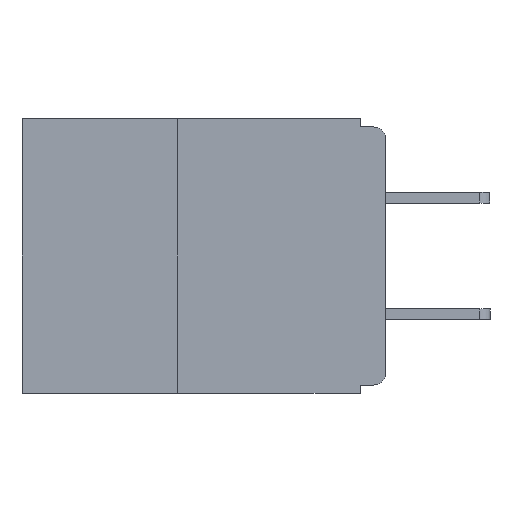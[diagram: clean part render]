
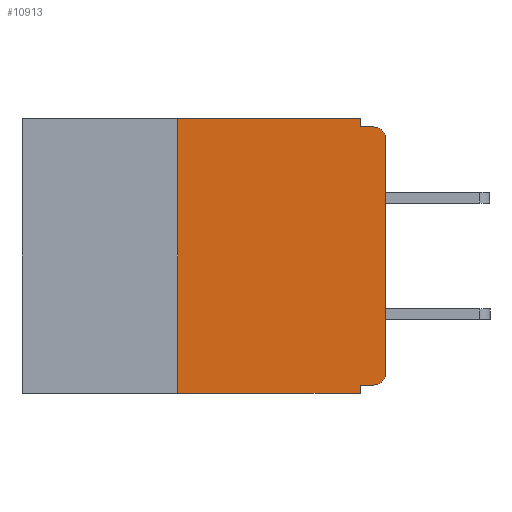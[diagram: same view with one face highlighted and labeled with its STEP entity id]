
A CAD part, left-side view. The second image highlights one B-rep face of the part: STEP entity #10913.
In plain terms, the highlighted planar face has unit normal (-1, 0, 0).
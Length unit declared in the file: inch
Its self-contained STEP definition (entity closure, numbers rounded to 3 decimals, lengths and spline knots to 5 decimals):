
#455 = CARTESIAN_POINT ( 'NONE',  ( 0., 0.437, -0.33 ) ) ;
#553 = VERTEX_POINT ( 'NONE', #17320 ) ;
#639 = CARTESIAN_POINT ( 'NONE',  ( 0., 0., -0.01 ) ) ;
#657 = CARTESIAN_POINT ( 'NONE',  ( 0., 0., -0.025 ) ) ;
#842 = CARTESIAN_POINT ( 'NONE',  ( 0., 0.031, 0. ) ) ;
#1207 = DIRECTION ( 'NONE',  ( 0., 0., -1. ) ) ;
#1218 = DIRECTION ( 'NONE',  ( 0., 0., -1. ) ) ;
#2066 = VECTOR ( 'NONE', #16568, 39.37008 ) ;
#2387 = EDGE_CURVE ( 'NONE', #8167, #9338, #11004, .T. ) ;
#2638 = CARTESIAN_POINT ( 'NONE',  ( 0., 0.25, 0. ) ) ;
#2918 = FACE_OUTER_BOUND ( 'NONE', #9005, .T. ) ;
#2960 = DIRECTION ( 'NONE',  ( 0., 0., -1. ) ) ;
#2979 = VERTEX_POINT ( 'NONE', #2638 ) ;
#2989 = VECTOR ( 'NONE', #12892, 39.37008 ) ;
#3006 = DIRECTION ( 'NONE',  ( 1., 0., 0. ) ) ;
#3076 = CARTESIAN_POINT ( 'NONE',  ( 0., 0.437, 0. ) ) ;
#3279 = PLANE ( 'NONE',  #16611 ) ;
#3420 = CARTESIAN_POINT ( 'NONE',  ( 0., 0.015, -0.01 ) ) ;
#3581 = CARTESIAN_POINT ( 'NONE',  ( 0., 0.031, -0.01 ) ) ;
#3980 = CARTESIAN_POINT ( 'NONE',  ( 0., 0., 0. ) ) ;
#4009 = VECTOR ( 'NONE', #13741, 39.37008 ) ;
#4166 = LINE ( 'NONE', #3980, #15136 ) ;
#4281 = DIRECTION ( 'NONE',  ( 0., 0., -1. ) ) ;
#4480 = DIRECTION ( 'NONE',  ( 0., -1., 0. ) ) ;
#4575 = EDGE_CURVE ( 'NONE', #5898, #14512, #12701, .T. ) ;
#4947 = ORIENTED_EDGE ( 'NONE', *, *, #17764, .F. ) ;
#5235 = VERTEX_POINT ( 'NONE', #3581 ) ;
#5738 = CARTESIAN_POINT ( 'NONE',  ( 0., 0.015, -0.32 ) ) ;
#5811 = DIRECTION ( 'NONE',  ( 0., 0., 1. ) ) ;
#5898 = VERTEX_POINT ( 'NONE', #657 ) ;
#6132 = VERTEX_POINT ( 'NONE', #16183 ) ;
#6234 = DIRECTION ( 'NONE',  ( 0., 0., -1. ) ) ;
#6428 = EDGE_CURVE ( 'NONE', #8167, #2979, #15448, .T. ) ;
#6537 = DIRECTION ( 'NONE',  ( -1., 0., 0. ) ) ;
#6635 = CARTESIAN_POINT ( 'NONE',  ( 0., 0.015, -0.025 ) ) ;
#6837 = ORIENTED_EDGE ( 'NONE', *, *, #17963, .F. ) ;
#6995 = LINE ( 'NONE', #12105, #2989 ) ;
#7040 = ORIENTED_EDGE ( 'NONE', *, *, #4575, .T. ) ;
#7387 = EDGE_CURVE ( 'NONE', #6132, #5235, #10359, .T. ) ;
#7752 = ORIENTED_EDGE ( 'NONE', *, *, #8477, .F. ) ;
#8167 = VERTEX_POINT ( 'NONE', #14017 ) ;
#8477 = EDGE_CURVE ( 'NONE', #14852, #12403, #6995, .T. ) ;
#8780 = CARTESIAN_POINT ( 'NONE',  ( 0., 0.031, -0.33 ) ) ;
#8935 = AXIS2_PLACEMENT_3D ( 'NONE', #6635, #6537, #6234 ) ;
#9005 = EDGE_LOOP ( 'NONE', ( #17293, #7040, #4947, #15885, #13090, #13534, #17111, #6837, #7752, #15242 ) ) ;
#9077 = EDGE_CURVE ( 'NONE', #553, #5898, #4166, .T. ) ;
#9338 = VERTEX_POINT ( 'NONE', #8780 ) ;
#10017 = DIRECTION ( 'NONE',  ( -1., 0., 0. ) ) ;
#10209 = CARTESIAN_POINT ( 'NONE',  ( 0., 0.437, 0. ) ) ;
#10359 = LINE ( 'NONE', #842, #17296 ) ;
#10363 = CARTESIAN_POINT ( 'NONE',  ( 0., 0.031, -0.32 ) ) ;
#10913 = ADVANCED_FACE ( 'NONE', ( #2918 ), #3279, .F. ) ;
#11004 = LINE ( 'NONE', #455, #13436 ) ;
#12105 = CARTESIAN_POINT ( 'NONE',  ( 0., 0., -0.32 ) ) ;
#12403 = VERTEX_POINT ( 'NONE', #10363 ) ;
#12448 = VECTOR ( 'NONE', #4480, 39.37008 ) ;
#12701 = CIRCLE ( 'NONE', #8935, 0.015 ) ;
#12892 = DIRECTION ( 'NONE',  ( 0., 1., 0. ) ) ;
#12941 = CARTESIAN_POINT ( 'NONE',  ( 0., 0.031, -0.33 ) ) ;
#13090 = ORIENTED_EDGE ( 'NONE', *, *, #15544, .F. ) ;
#13436 = VECTOR ( 'NONE', #16319, 39.37008 ) ;
#13466 = VECTOR ( 'NONE', #4281, 39.37008 ) ;
#13534 = ORIENTED_EDGE ( 'NONE', *, *, #6428, .F. ) ;
#13615 = CARTESIAN_POINT ( 'NONE',  ( 0., 0.25, -0.33 ) ) ;
#13741 = DIRECTION ( 'NONE',  ( 0., 0., 1. ) ) ;
#14017 = CARTESIAN_POINT ( 'NONE',  ( 0., 0.25, -0.33 ) ) ;
#14190 = CIRCLE ( 'NONE', #16413, 0.015 ) ;
#14512 = VERTEX_POINT ( 'NONE', #3420 ) ;
#14852 = VERTEX_POINT ( 'NONE', #5738 ) ;
#15136 = VECTOR ( 'NONE', #5811, 39.37008 ) ;
#15242 = ORIENTED_EDGE ( 'NONE', *, *, #15473, .T. ) ;
#15448 = LINE ( 'NONE', #13615, #4009 ) ;
#15473 = EDGE_CURVE ( 'NONE', #14852, #553, #14190, .T. ) ;
#15544 = EDGE_CURVE ( 'NONE', #2979, #6132, #16103, .T. ) ;
#15885 = ORIENTED_EDGE ( 'NONE', *, *, #7387, .F. ) ;
#16103 = LINE ( 'NONE', #10209, #12448 ) ;
#16183 = CARTESIAN_POINT ( 'NONE',  ( 0., 0.031, 0. ) ) ;
#16226 = LINE ( 'NONE', #12941, #13466 ) ;
#16319 = DIRECTION ( 'NONE',  ( 0., -1., 0. ) ) ;
#16413 = AXIS2_PLACEMENT_3D ( 'NONE', #18255, #10017, #1207 ) ;
#16568 = DIRECTION ( 'NONE',  ( 0., -1., 0. ) ) ;
#16611 = AXIS2_PLACEMENT_3D ( 'NONE', #3076, #3006, #2960 ) ;
#16853 = LINE ( 'NONE', #639, #2066 ) ;
#17111 = ORIENTED_EDGE ( 'NONE', *, *, #2387, .T. ) ;
#17293 = ORIENTED_EDGE ( 'NONE', *, *, #9077, .T. ) ;
#17296 = VECTOR ( 'NONE', #1218, 39.37008 ) ;
#17320 = CARTESIAN_POINT ( 'NONE',  ( 0., 0., -0.305 ) ) ;
#17764 = EDGE_CURVE ( 'NONE', #5235, #14512, #16853, .T. ) ;
#17963 = EDGE_CURVE ( 'NONE', #12403, #9338, #16226, .T. ) ;
#18255 = CARTESIAN_POINT ( 'NONE',  ( 0., 0.015, -0.305 ) ) ;
